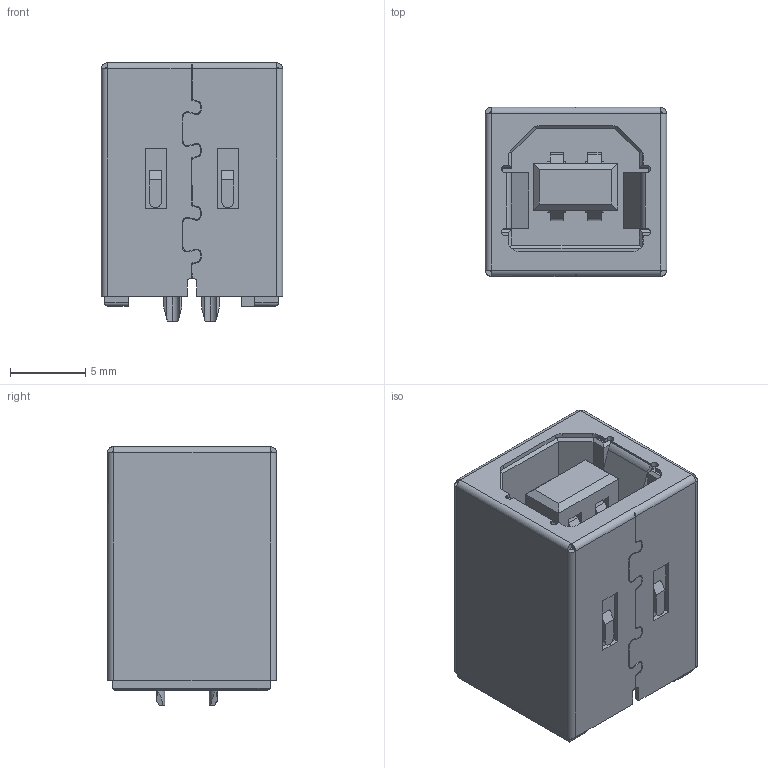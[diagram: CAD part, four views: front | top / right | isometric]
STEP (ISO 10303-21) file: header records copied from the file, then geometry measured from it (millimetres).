
FILE_DESCRIPTION (( 'STEP AP214' ), '1' );
FILE_NAME ('690S204-190-221.STEP', '2021-01-14T21:34:30', ( '' ), ( '' ), 'SwSTEP 2.0', 'SolidWorks 2020', '' );
FILE_SCHEMA (( 'AUTOMOTIVE_DESIGN' ));
Length unit declared in the file: millimetre
Products named in the file (4): 690S204-190-221; Insulator 690S204-X90-22X_Black; Contact 690S204-X90-22X; Shell 690S204-X90-22X
Assembly tree (6 placements, depth 2):
  690S204-190-221
    Insulator 690S204-X90-22X_Black
    Contact 690S204-X90-22X  x4
    Shell 690S204-X90-22X
Bounding box: 12.04 x 11.2 x 17.15 mm (x, y, z)
Volume: 1363 mm3; surface area: 3376.6 mm2
Topology: 6 solids, 6 shells, 629 faces, 1794 edges, 1166 vertices
Faces by surface type: plane 428, cylinder 201
Entity records: 16198 total; most frequent: CARTESIAN_POINT 2920, ORIENTED_EDGE 2838, DIRECTION 2680, EDGE_CURVE 1419, LINE 1100, VECTOR 1100, VERTEX_POINT 926, AXIS2_PLACEMENT_3D 790
